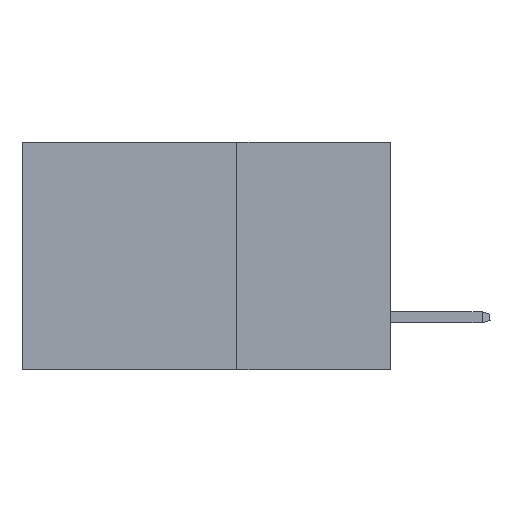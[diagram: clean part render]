
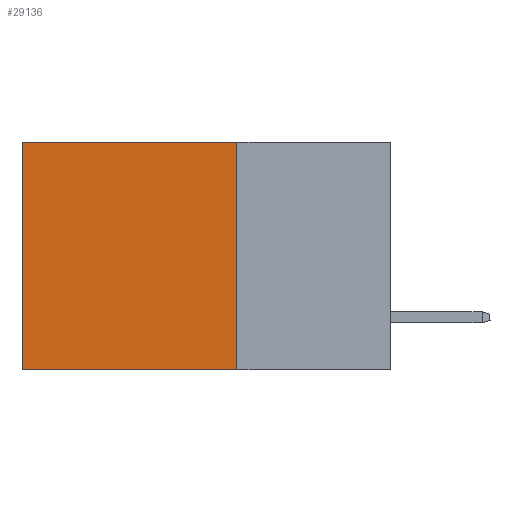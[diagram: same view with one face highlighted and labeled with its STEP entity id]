
A CAD part, left-side view. The second image highlights one B-rep face of the part: STEP entity #29136.
In plain terms, the highlighted planar face has unit normal (-1, 0, 0).
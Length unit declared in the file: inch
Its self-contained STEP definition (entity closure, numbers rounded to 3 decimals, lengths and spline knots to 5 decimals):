
#32 = EDGE_LOOP ( 'NONE', ( #3008, #12692, #11573, #2427 ) ) ;
#1017 = VECTOR ( 'NONE', #3161, 39.37008 ) ;
#1608 = DIRECTION ( 'NONE',  ( 0., 1., 0. ) ) ;
#2427 = ORIENTED_EDGE ( 'NONE', *, *, #25183, .T. ) ;
#2604 = EDGE_CURVE ( 'NONE', #10682, #12889, #29858, .T. ) ;
#2828 = DIRECTION ( 'NONE',  ( 0., 0., -1. ) ) ;
#3008 = ORIENTED_EDGE ( 'NONE', *, *, #2604, .T. ) ;
#3161 = DIRECTION ( 'NONE',  ( 0., 1., 0. ) ) ;
#3528 = VECTOR ( 'NONE', #2828, 39.37008 ) ;
#4103 = CARTESIAN_POINT ( 'NONE',  ( 0.2875, 0.25, 0. ) ) ;
#4272 = VERTEX_POINT ( 'NONE', #7720 ) ;
#6929 = CARTESIAN_POINT ( 'NONE',  ( 0.2875, 0.25, 0. ) ) ;
#7484 = VECTOR ( 'NONE', #1608, 39.37008 ) ;
#7720 = CARTESIAN_POINT ( 'NONE',  ( 0.2875, 0.25, -0.37 ) ) ;
#9737 = CARTESIAN_POINT ( 'NONE',  ( 0.2875, 0.25, 0. ) ) ;
#10359 = EDGE_CURVE ( 'NONE', #4272, #12889, #15268, .T. ) ;
#10682 = VERTEX_POINT ( 'NONE', #21523 ) ;
#10940 = FACE_OUTER_BOUND ( 'NONE', #32, .T. ) ;
#11573 = ORIENTED_EDGE ( 'NONE', *, *, #28624, .F. ) ;
#12502 = PLANE ( 'NONE',  #20027 ) ;
#12692 = ORIENTED_EDGE ( 'NONE', *, *, #10359, .F. ) ;
#12889 = VERTEX_POINT ( 'NONE', #24253 ) ;
#15268 = LINE ( 'NONE', #30937, #1017 ) ;
#19805 = VECTOR ( 'NONE', #34708, 39.37008 ) ;
#20027 = AXIS2_PLACEMENT_3D ( 'NONE', #9737, #35083, #20811 ) ;
#20811 = DIRECTION ( 'NONE',  ( 0., 0., -1. ) ) ;
#21141 = CARTESIAN_POINT ( 'NONE',  ( 0.2875, 0.6, 0. ) ) ;
#21523 = CARTESIAN_POINT ( 'NONE',  ( 0.2875, 0.6, 0. ) ) ;
#23925 = LINE ( 'NONE', #6929, #7484 ) ;
#23999 = VERTEX_POINT ( 'NONE', #4103 ) ;
#24253 = CARTESIAN_POINT ( 'NONE',  ( 0.2875, 0.6, -0.37 ) ) ;
#25183 = EDGE_CURVE ( 'NONE', #23999, #10682, #23925, .T. ) ;
#27398 = LINE ( 'NONE', #32226, #3528 ) ;
#28624 = EDGE_CURVE ( 'NONE', #23999, #4272, #27398, .T. ) ;
#29136 = ADVANCED_FACE ( 'NONE', ( #10940 ), #12502, .F. ) ;
#29858 = LINE ( 'NONE', #21141, #19805 ) ;
#30937 = CARTESIAN_POINT ( 'NONE',  ( 0.2875, 0.25, -0.37 ) ) ;
#32226 = CARTESIAN_POINT ( 'NONE',  ( 0.2875, 0.25, 0. ) ) ;
#34708 = DIRECTION ( 'NONE',  ( 0., 0., -1. ) ) ;
#35083 = DIRECTION ( 'NONE',  ( 1., 0., 0. ) ) ;
